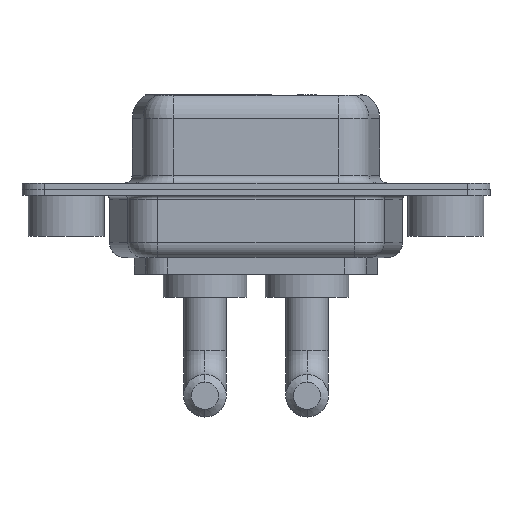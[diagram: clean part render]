
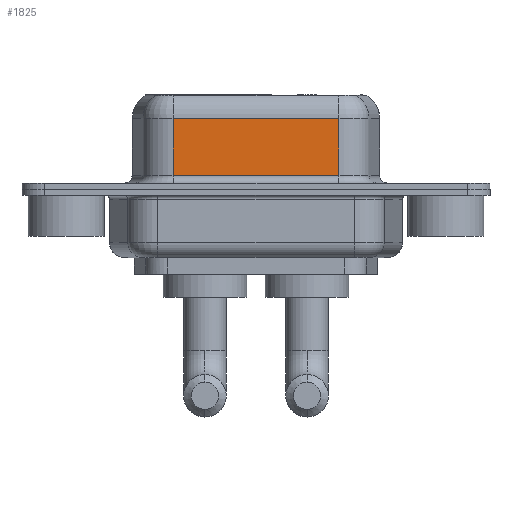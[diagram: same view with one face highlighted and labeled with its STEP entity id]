
A CAD part, front view. The second image highlights one B-rep face of the part: STEP entity #1825.
In plain terms, the highlighted planar face has unit normal (0, -1, 0).
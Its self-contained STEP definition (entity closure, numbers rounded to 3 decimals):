
#265 = VECTOR ( 'NONE', #6368, 1000. ) ;
#1220 = VERTEX_POINT ( 'NONE', #10524 ) ;
#1271 = DIRECTION ( 'NONE',  ( -1., 0., 0. ) ) ;
#1342 = CARTESIAN_POINT ( 'NONE',  ( 17.962, -3.95, 6.4 ) ) ;
#1825 = ADVANCED_FACE ( 'NONE', ( #2423 ), #12578, .F. ) ;
#1962 = VERTEX_POINT ( 'NONE', #12903 ) ;
#2423 = FACE_OUTER_BOUND ( 'NONE', #7110, .T. ) ;
#2681 = ORIENTED_EDGE ( 'NONE', *, *, #11374, .T. ) ;
#2744 = ORIENTED_EDGE ( 'NONE', *, *, #5870, .T. ) ;
#3054 = CARTESIAN_POINT ( 'NONE',  ( 7.038, -3.95, 6.4 ) ) ;
#3326 = DIRECTION ( 'NONE',  ( 1., 0., 0. ) ) ;
#3391 = VECTOR ( 'NONE', #3326, 1000. ) ;
#3595 = CARTESIAN_POINT ( 'NONE',  ( 7.038, -3.95, 4.65 ) ) ;
#3776 = ORIENTED_EDGE ( 'NONE', *, *, #7347, .T. ) ;
#5079 = EDGE_CURVE ( 'NONE', #1962, #1220, #10626, .T. ) ;
#5785 = VECTOR ( 'NONE', #10295, 1000. ) ;
#5870 = EDGE_CURVE ( 'NONE', #10159, #6353, #13329, .T. ) ;
#6353 = VERTEX_POINT ( 'NONE', #8641 ) ;
#6368 = DIRECTION ( 'NONE',  ( 0., 0., -1. ) ) ;
#7110 = EDGE_LOOP ( 'NONE', ( #13334, #2681, #2744, #3776 ) ) ;
#7347 = EDGE_CURVE ( 'NONE', #6353, #1220, #9487, .T. ) ;
#7718 = VECTOR ( 'NONE', #11682, 1000. ) ;
#8636 = CARTESIAN_POINT ( 'NONE',  ( 17.962, -3.95, 4.65 ) ) ;
#8641 = CARTESIAN_POINT ( 'NONE',  ( 7.038, -3.95, 0.9 ) ) ;
#9487 = LINE ( 'NONE', #11651, #3391 ) ;
#9663 = DIRECTION ( 'NONE',  ( 0., 1., 0. ) ) ;
#10159 = VERTEX_POINT ( 'NONE', #3595 ) ;
#10295 = DIRECTION ( 'NONE',  ( 0., 0., -1. ) ) ;
#10524 = CARTESIAN_POINT ( 'NONE',  ( 17.962, -3.95, 0.9 ) ) ;
#10554 = CARTESIAN_POINT ( 'NONE',  ( 17.962, -3.95, 6.4 ) ) ;
#10626 = LINE ( 'NONE', #1342, #265 ) ;
#11205 = AXIS2_PLACEMENT_3D ( 'NONE', #10554, #9663, #1271 ) ;
#11374 = EDGE_CURVE ( 'NONE', #1962, #10159, #12367, .T. ) ;
#11651 = CARTESIAN_POINT ( 'NONE',  ( 17.962, -3.95, 0.9 ) ) ;
#11682 = DIRECTION ( 'NONE',  ( -1., 0., 0. ) ) ;
#12367 = LINE ( 'NONE', #8636, #7718 ) ;
#12578 = PLANE ( 'NONE',  #11205 ) ;
#12903 = CARTESIAN_POINT ( 'NONE',  ( 17.962, -3.95, 4.65 ) ) ;
#13329 = LINE ( 'NONE', #3054, #5785 ) ;
#13334 = ORIENTED_EDGE ( 'NONE', *, *, #5079, .F. ) ;
